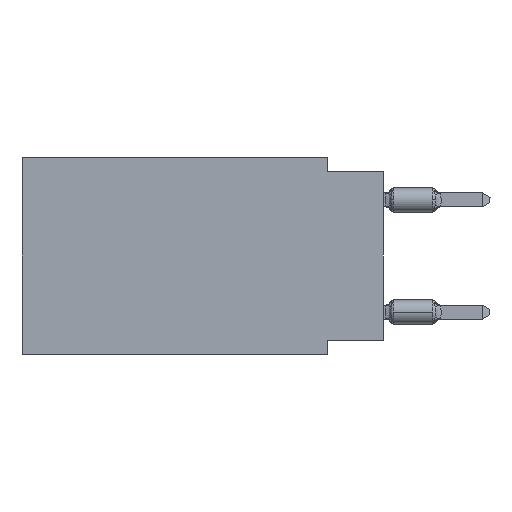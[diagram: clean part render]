
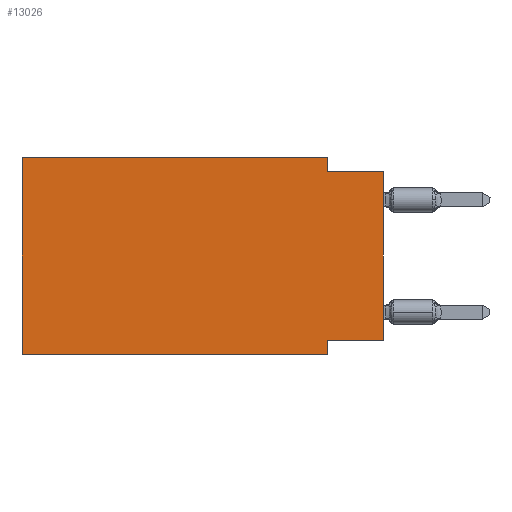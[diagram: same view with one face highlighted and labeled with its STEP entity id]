
A CAD part, left-side view. The second image highlights one B-rep face of the part: STEP entity #13026.
In plain terms, the highlighted planar face has unit normal (-1, 0, 0).
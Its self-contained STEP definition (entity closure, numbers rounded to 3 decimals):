
#883 = CARTESIAN_POINT ( 'NONE',  ( 0., 0., -0.635 ) ) ;
#930 = PLANE ( 'NONE',  #15291 ) ;
#1968 = DIRECTION ( 'NONE',  ( 0., 0., 1. ) ) ;
#3401 = VECTOR ( 'NONE', #3942, 1000. ) ;
#3942 = DIRECTION ( 'NONE',  ( 0., 0., -1. ) ) ;
#4552 = ORIENTED_EDGE ( 'NONE', *, *, #60283, .F. ) ;
#4845 = FACE_OUTER_BOUND ( 'NONE', #50685, .T. ) ;
#5265 = CARTESIAN_POINT ( 'NONE',  ( 0., 2.54, 0. ) ) ;
#7675 = EDGE_CURVE ( 'NONE', #61579, #59427, #61696, .T. ) ;
#7749 = ORIENTED_EDGE ( 'NONE', *, *, #7675, .T. ) ;
#8304 = CARTESIAN_POINT ( 'NONE',  ( 0., 16.383, 0. ) ) ;
#9563 = CARTESIAN_POINT ( 'NONE',  ( 0., 0., -0.635 ) ) ;
#11169 = VERTEX_POINT ( 'NONE', #37594 ) ;
#12969 = ORIENTED_EDGE ( 'NONE', *, *, #16263, .F. ) ;
#13026 = ADVANCED_FACE ( 'NONE', ( #4845 ), #930, .F. ) ;
#14391 = LINE ( 'NONE', #60049, #3401 ) ;
#15291 = AXIS2_PLACEMENT_3D ( 'NONE', #19891, #25747, #45625 ) ;
#15746 = VERTEX_POINT ( 'NONE', #56779 ) ;
#16009 = VECTOR ( 'NONE', #1968, 1000. ) ;
#16263 = EDGE_CURVE ( 'NONE', #15746, #48179, #17172, .T. ) ;
#17172 = LINE ( 'NONE', #62489, #26015 ) ;
#17397 = VECTOR ( 'NONE', #27370, 1000. ) ;
#17487 = DIRECTION ( 'NONE',  ( 0., 0., 1. ) ) ;
#19674 = CARTESIAN_POINT ( 'NONE',  ( 0., 2.54, -8.89 ) ) ;
#19859 = EDGE_CURVE ( 'NONE', #48179, #39973, #33423, .T. ) ;
#19891 = CARTESIAN_POINT ( 'NONE',  ( 0., 16.383, 0. ) ) ;
#20506 = EDGE_CURVE ( 'NONE', #11169, #63917, #14391, .T. ) ;
#20621 = ORIENTED_EDGE ( 'NONE', *, *, #20506, .F. ) ;
#21518 = CARTESIAN_POINT ( 'NONE',  ( 0., 16.383, -8.89 ) ) ;
#21839 = CARTESIAN_POINT ( 'NONE',  ( 0., 0., -8.255 ) ) ;
#23353 = DIRECTION ( 'NONE',  ( 0., 1., 0. ) ) ;
#23956 = DIRECTION ( 'NONE',  ( 0., -1., 0. ) ) ;
#25702 = LINE ( 'NONE', #883, #63478 ) ;
#25747 = DIRECTION ( 'NONE',  ( 1., 0., 0. ) ) ;
#26015 = VECTOR ( 'NONE', #17487, 1000. ) ;
#27370 = DIRECTION ( 'NONE',  ( 0., -1., 0. ) ) ;
#28042 = EDGE_CURVE ( 'NONE', #15746, #63917, #42020, .T. ) ;
#29610 = DIRECTION ( 'NONE',  ( 0., 0., -1. ) ) ;
#31000 = EDGE_CURVE ( 'NONE', #61579, #11169, #52376, .T. ) ;
#31463 = VECTOR ( 'NONE', #23353, 1000. ) ;
#33423 = LINE ( 'NONE', #37665, #41912 ) ;
#33637 = ORIENTED_EDGE ( 'NONE', *, *, #19859, .F. ) ;
#33770 = CARTESIAN_POINT ( 'NONE',  ( 0., 0., -8.255 ) ) ;
#35135 = CARTESIAN_POINT ( 'NONE',  ( 0., 2.54, 0. ) ) ;
#37084 = ORIENTED_EDGE ( 'NONE', *, *, #31000, .F. ) ;
#37594 = CARTESIAN_POINT ( 'NONE',  ( 0., 2.54, -8.255 ) ) ;
#37665 = CARTESIAN_POINT ( 'NONE',  ( 0., 16.383, 0. ) ) ;
#39059 = EDGE_CURVE ( 'NONE', #39973, #63034, #39690, .T. ) ;
#39302 = VECTOR ( 'NONE', #29610, 1000. ) ;
#39690 = LINE ( 'NONE', #35135, #39302 ) ;
#39973 = VERTEX_POINT ( 'NONE', #5265 ) ;
#41912 = VECTOR ( 'NONE', #23956, 1000. ) ;
#42020 = LINE ( 'NONE', #21518, #17397 ) ;
#42103 = ORIENTED_EDGE ( 'NONE', *, *, #39059, .F. ) ;
#42354 = CARTESIAN_POINT ( 'NONE',  ( 0., 2.54, -0.635 ) ) ;
#45579 = DIRECTION ( 'NONE',  ( 0., -1., 0. ) ) ;
#45625 = DIRECTION ( 'NONE',  ( 0., 0., -1. ) ) ;
#48179 = VERTEX_POINT ( 'NONE', #8304 ) ;
#50685 = EDGE_LOOP ( 'NONE', ( #7749, #4552, #42103, #33637, #12969, #54934, #20621, #37084 ) ) ;
#52376 = LINE ( 'NONE', #33770, #31463 ) ;
#54934 = ORIENTED_EDGE ( 'NONE', *, *, #28042, .T. ) ;
#56779 = CARTESIAN_POINT ( 'NONE',  ( 0., 16.383, -8.89 ) ) ;
#59427 = VERTEX_POINT ( 'NONE', #9563 ) ;
#60049 = CARTESIAN_POINT ( 'NONE',  ( 0., 2.54, -8.89 ) ) ;
#60283 = EDGE_CURVE ( 'NONE', #63034, #59427, #25702, .T. ) ;
#61052 = CARTESIAN_POINT ( 'NONE',  ( 0., 0., 0. ) ) ;
#61579 = VERTEX_POINT ( 'NONE', #21839 ) ;
#61696 = LINE ( 'NONE', #61052, #16009 ) ;
#62489 = CARTESIAN_POINT ( 'NONE',  ( 0., 16.383, 0. ) ) ;
#63034 = VERTEX_POINT ( 'NONE', #42354 ) ;
#63478 = VECTOR ( 'NONE', #45579, 1000. ) ;
#63917 = VERTEX_POINT ( 'NONE', #19674 ) ;
